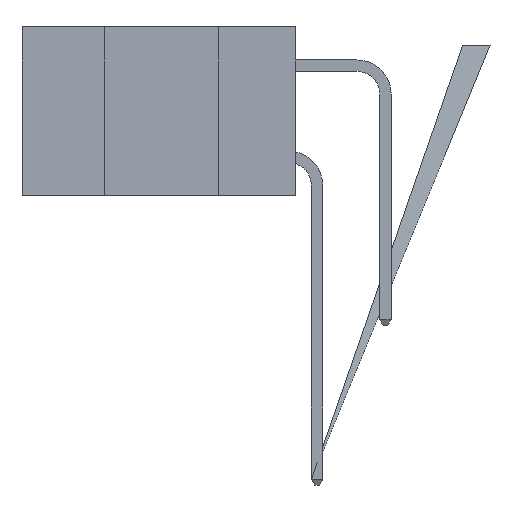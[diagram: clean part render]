
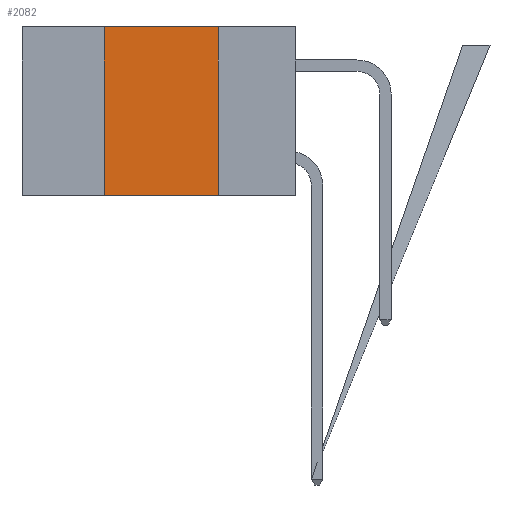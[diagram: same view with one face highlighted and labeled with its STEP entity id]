
A CAD part, left-side view. The second image highlights one B-rep face of the part: STEP entity #2082.
In plain terms, the highlighted planar face has unit normal (-1, 0, 0).
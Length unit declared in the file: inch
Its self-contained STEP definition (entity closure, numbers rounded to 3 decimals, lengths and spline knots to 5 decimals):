
#268 = CARTESIAN_POINT ( 'NONE',  ( 0., 0.42, 0. ) ) ;
#1328 = VERTEX_POINT ( 'NONE', #268 ) ;
#1858 = VERTEX_POINT ( 'NONE', #12112 ) ;
#1889 = EDGE_CURVE ( 'NONE', #7153, #1328, #5637, .T. ) ;
#2082 = ADVANCED_FACE ( 'NONE', ( #3168 ), #7607, .F. ) ;
#2489 = CARTESIAN_POINT ( 'NONE',  ( 0., 0.42, -0.37 ) ) ;
#3168 = FACE_OUTER_BOUND ( 'NONE', #9381, .T. ) ;
#3784 = LINE ( 'NONE', #11059, #5851 ) ;
#3985 = ORIENTED_EDGE ( 'NONE', *, *, #5556, .F. ) ;
#4012 = ORIENTED_EDGE ( 'NONE', *, *, #4923, .F. ) ;
#4115 = CARTESIAN_POINT ( 'NONE',  ( 0., 0.17, 0. ) ) ;
#4133 = DIRECTION ( 'NONE',  ( 0., 0., -1. ) ) ;
#4923 = EDGE_CURVE ( 'NONE', #1328, #1858, #5596, .T. ) ;
#5388 = DIRECTION ( 'NONE',  ( 0., -1., 0. ) ) ;
#5556 = EDGE_CURVE ( 'NONE', #1858, #9246, #12299, .T. ) ;
#5596 = LINE ( 'NONE', #10835, #10712 ) ;
#5615 = DIRECTION ( 'NONE',  ( 0., -1., 0. ) ) ;
#5637 = LINE ( 'NONE', #8266, #9855 ) ;
#5761 = CARTESIAN_POINT ( 'NONE',  ( 0., 0.17, -0.37 ) ) ;
#5851 = VECTOR ( 'NONE', #5615, 39.37008 ) ;
#6242 = ORIENTED_EDGE ( 'NONE', *, *, #1889, .F. ) ;
#6692 = ORIENTED_EDGE ( 'NONE', *, *, #8190, .T. ) ;
#7153 = VERTEX_POINT ( 'NONE', #2489 ) ;
#7177 = DIRECTION ( 'NONE',  ( 0., 0., 1. ) ) ;
#7587 = DIRECTION ( 'NONE',  ( 1., 0., 0. ) ) ;
#7607 = PLANE ( 'NONE',  #10650 ) ;
#7695 = CARTESIAN_POINT ( 'NONE',  ( 0., 0.6, 0. ) ) ;
#8190 = EDGE_CURVE ( 'NONE', #7153, #9246, #3784, .T. ) ;
#8266 = CARTESIAN_POINT ( 'NONE',  ( 0., 0.42, 0. ) ) ;
#9246 = VERTEX_POINT ( 'NONE', #5761 ) ;
#9381 = EDGE_LOOP ( 'NONE', ( #3985, #4012, #6242, #6692 ) ) ;
#9855 = VECTOR ( 'NONE', #7177, 39.37008 ) ;
#10650 = AXIS2_PLACEMENT_3D ( 'NONE', #7695, #7587, #4133 ) ;
#10712 = VECTOR ( 'NONE', #5388, 39.37008 ) ;
#10835 = CARTESIAN_POINT ( 'NONE',  ( 0., 0.6, 0. ) ) ;
#11059 = CARTESIAN_POINT ( 'NONE',  ( 0., 0.6, -0.37 ) ) ;
#12008 = VECTOR ( 'NONE', #12485, 39.37008 ) ;
#12112 = CARTESIAN_POINT ( 'NONE',  ( 0., 0.17, 0. ) ) ;
#12299 = LINE ( 'NONE', #4115, #12008 ) ;
#12485 = DIRECTION ( 'NONE',  ( 0., 0., -1. ) ) ;
